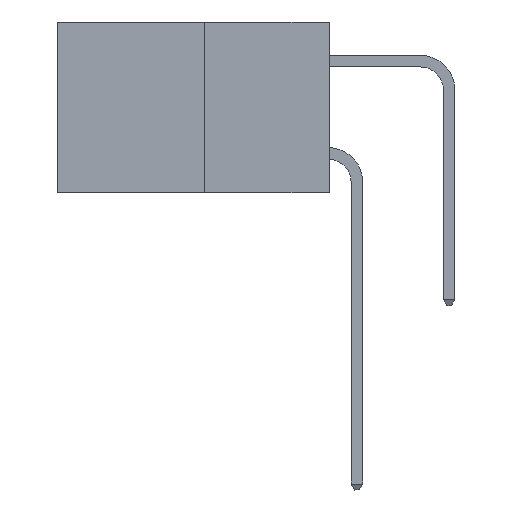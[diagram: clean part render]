
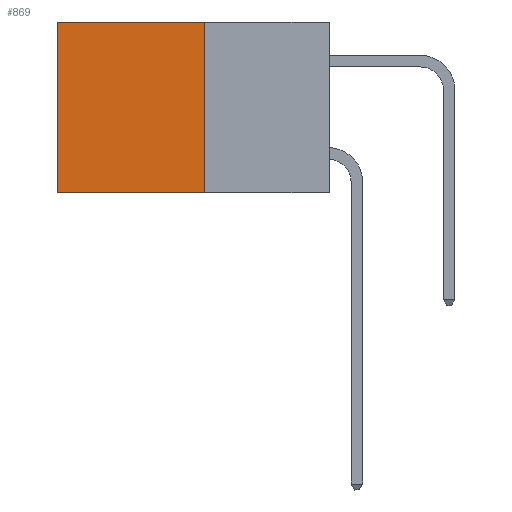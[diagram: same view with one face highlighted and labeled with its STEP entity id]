
A CAD part, left-side view. The second image highlights one B-rep face of the part: STEP entity #869.
In plain terms, the highlighted planar face has unit normal (-1, 0, 0).
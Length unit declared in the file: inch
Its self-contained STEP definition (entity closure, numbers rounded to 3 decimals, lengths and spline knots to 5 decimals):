
#338 = ORIENTED_EDGE ( 'NONE', *, *, #16536, .T. ) ;
#869 = ADVANCED_FACE ( 'NONE', ( #14040 ), #6617, .F. ) ;
#1138 = ORIENTED_EDGE ( 'NONE', *, *, #11023, .T. ) ;
#1264 = VECTOR ( 'NONE', #8459, 39.37008 ) ;
#1961 = ORIENTED_EDGE ( 'NONE', *, *, #6528, .F. ) ;
#2726 = CARTESIAN_POINT ( 'NONE',  ( 0.277, 0.27, -0.37 ) ) ;
#3036 = AXIS2_PLACEMENT_3D ( 'NONE', #9308, #9453, #17103 ) ;
#3172 = CARTESIAN_POINT ( 'NONE',  ( 0.277, 0.27, 0. ) ) ;
#3463 = VERTEX_POINT ( 'NONE', #8717 ) ;
#3684 = VERTEX_POINT ( 'NONE', #13752 ) ;
#3989 = CARTESIAN_POINT ( 'NONE',  ( 0.277, 0.59, -0.37 ) ) ;
#4154 = VECTOR ( 'NONE', #17185, 39.37008 ) ;
#4529 = LINE ( 'NONE', #2726, #11863 ) ;
#4586 = LINE ( 'NONE', #6984, #1264 ) ;
#5715 = CARTESIAN_POINT ( 'NONE',  ( 0.277, 0.59, -0.37 ) ) ;
#6528 = EDGE_CURVE ( 'NONE', #3463, #15081, #4529, .T. ) ;
#6535 = EDGE_LOOP ( 'NONE', ( #338, #1961, #10773, #1138 ) ) ;
#6617 = PLANE ( 'NONE',  #3036 ) ;
#6984 = CARTESIAN_POINT ( 'NONE',  ( 0.277, 0.27, -0.37 ) ) ;
#7767 = VERTEX_POINT ( 'NONE', #3172 ) ;
#8459 = DIRECTION ( 'NONE',  ( 0., 0., -1. ) ) ;
#8549 = DIRECTION ( 'NONE',  ( 0., 1., 0. ) ) ;
#8556 = LINE ( 'NONE', #5715, #4154 ) ;
#8717 = CARTESIAN_POINT ( 'NONE',  ( 0.277, 0.27, -0.37 ) ) ;
#9308 = CARTESIAN_POINT ( 'NONE',  ( 0.277, 0.27, -0.37 ) ) ;
#9453 = DIRECTION ( 'NONE',  ( 1., 0., 0. ) ) ;
#10383 = LINE ( 'NONE', #13407, #17897 ) ;
#10773 = ORIENTED_EDGE ( 'NONE', *, *, #12060, .F. ) ;
#11023 = EDGE_CURVE ( 'NONE', #7767, #3684, #10383, .T. ) ;
#11863 = VECTOR ( 'NONE', #8549, 39.37008 ) ;
#12060 = EDGE_CURVE ( 'NONE', #7767, #3463, #4586, .T. ) ;
#13407 = CARTESIAN_POINT ( 'NONE',  ( 0.277, 0.27, 0. ) ) ;
#13752 = CARTESIAN_POINT ( 'NONE',  ( 0.277, 0.59, 0. ) ) ;
#14040 = FACE_OUTER_BOUND ( 'NONE', #6535, .T. ) ;
#14819 = DIRECTION ( 'NONE',  ( 0., 1., 0. ) ) ;
#15081 = VERTEX_POINT ( 'NONE', #3989 ) ;
#16536 = EDGE_CURVE ( 'NONE', #3684, #15081, #8556, .T. ) ;
#17103 = DIRECTION ( 'NONE',  ( 0., 0., -1. ) ) ;
#17185 = DIRECTION ( 'NONE',  ( 0., 0., -1. ) ) ;
#17897 = VECTOR ( 'NONE', #14819, 39.37008 ) ;
